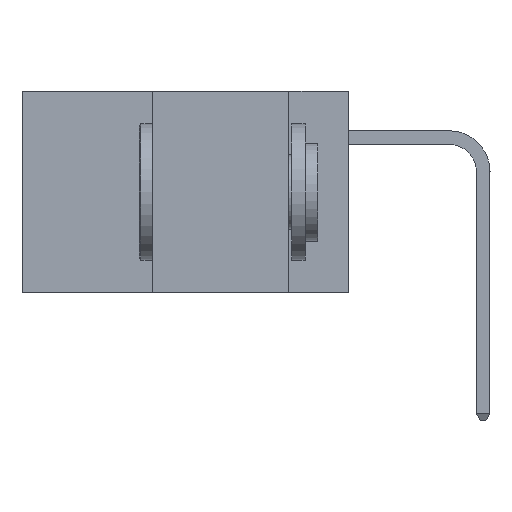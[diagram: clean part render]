
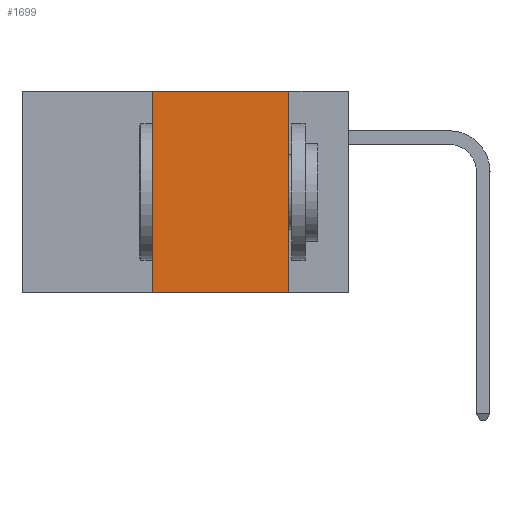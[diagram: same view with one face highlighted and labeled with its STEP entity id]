
A CAD part, left-side view. The second image highlights one B-rep face of the part: STEP entity #1699.
In plain terms, the highlighted planar face has unit normal (-1, 0, 0).
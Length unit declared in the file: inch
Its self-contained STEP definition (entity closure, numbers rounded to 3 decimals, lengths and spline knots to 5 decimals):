
#1378 = VECTOR ( 'NONE', #38266, 39.37008 ) ;
#1699 = ADVANCED_FACE ( 'NONE', ( #29781 ), #10970, .F. ) ;
#2855 = CARTESIAN_POINT ( 'NONE',  ( 0., 0.6, 0. ) ) ;
#3693 = EDGE_CURVE ( 'NONE', #9828, #48625, #48693, .T. ) ;
#4793 = LINE ( 'NONE', #6548, #37878 ) ;
#5894 = EDGE_LOOP ( 'NONE', ( #12435, #25477, #21144, #48051 ) ) ;
#6548 = CARTESIAN_POINT ( 'NONE',  ( 0., 0.11, 0. ) ) ;
#9828 = VERTEX_POINT ( 'NONE', #33523 ) ;
#10970 = PLANE ( 'NONE',  #45215 ) ;
#12244 = DIRECTION ( 'NONE',  ( 0., 0., 1. ) ) ;
#12435 = ORIENTED_EDGE ( 'NONE', *, *, #36569, .F. ) ;
#13861 = CARTESIAN_POINT ( 'NONE',  ( 0., 0.11, 0. ) ) ;
#13936 = DIRECTION ( 'NONE',  ( 0., -1., 0. ) ) ;
#15142 = VERTEX_POINT ( 'NONE', #26570 ) ;
#18336 = DIRECTION ( 'NONE',  ( 0., 0., -1. ) ) ;
#20058 = LINE ( 'NONE', #26367, #1378 ) ;
#21144 = ORIENTED_EDGE ( 'NONE', *, *, #45382, .F. ) ;
#25477 = ORIENTED_EDGE ( 'NONE', *, *, #43360, .F. ) ;
#26079 = DIRECTION ( 'NONE',  ( 1., 0., 0. ) ) ;
#26367 = CARTESIAN_POINT ( 'NONE',  ( 0., 0.6, 0. ) ) ;
#26570 = CARTESIAN_POINT ( 'NONE',  ( 0., 0.36, 0. ) ) ;
#28432 = VERTEX_POINT ( 'NONE', #13861 ) ;
#29386 = LINE ( 'NONE', #34899, #34250 ) ;
#29781 = FACE_OUTER_BOUND ( 'NONE', #5894, .T. ) ;
#33523 = CARTESIAN_POINT ( 'NONE',  ( 0., 0.36, -0.37 ) ) ;
#34018 = CARTESIAN_POINT ( 'NONE',  ( 0., 0.11, -0.37 ) ) ;
#34250 = VECTOR ( 'NONE', #12244, 39.37008 ) ;
#34899 = CARTESIAN_POINT ( 'NONE',  ( 0., 0.36, 0. ) ) ;
#36569 = EDGE_CURVE ( 'NONE', #28432, #48625, #4793, .T. ) ;
#37878 = VECTOR ( 'NONE', #18336, 39.37008 ) ;
#37981 = DIRECTION ( 'NONE',  ( 0., 0., -1. ) ) ;
#38266 = DIRECTION ( 'NONE',  ( 0., -1., 0. ) ) ;
#43360 = EDGE_CURVE ( 'NONE', #15142, #28432, #20058, .T. ) ;
#44258 = CARTESIAN_POINT ( 'NONE',  ( 0., 0.6, -0.37 ) ) ;
#45109 = VECTOR ( 'NONE', #13936, 39.37008 ) ;
#45215 = AXIS2_PLACEMENT_3D ( 'NONE', #2855, #26079, #37981 ) ;
#45382 = EDGE_CURVE ( 'NONE', #9828, #15142, #29386, .T. ) ;
#48051 = ORIENTED_EDGE ( 'NONE', *, *, #3693, .T. ) ;
#48625 = VERTEX_POINT ( 'NONE', #34018 ) ;
#48693 = LINE ( 'NONE', #44258, #45109 ) ;
